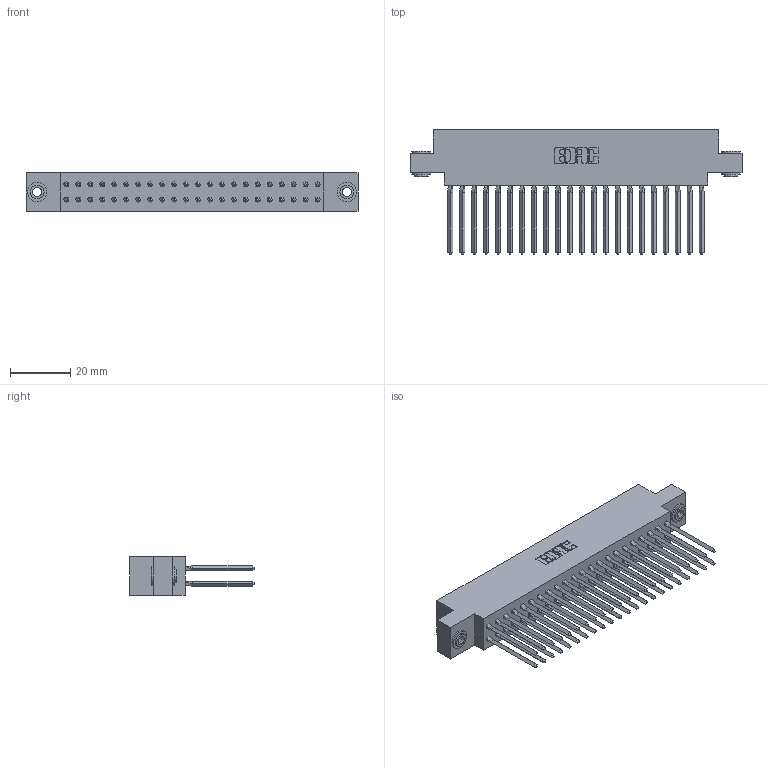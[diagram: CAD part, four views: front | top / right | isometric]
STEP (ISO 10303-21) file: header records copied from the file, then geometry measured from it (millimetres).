
FILE_DESCRIPTION (( 'STEP AP203' ), '1' );
FILE_NAME ('317-044-543-803.STEP', '2020-02-28T02:12:42', ( '' ), ( '' ), 'SwSTEP 2.0', 'SolidWorks 2016', '' );
FILE_SCHEMA (( 'CONFIG_CONTROL_DESIGN' ));
Length unit declared in the file: inch
Products named in the file (4): 317-290-001_543; 317-044-543-803; 345-250-002_345-250-002-102; 317 Part_.156 Dia - TH
Assembly tree (47 placements, depth 2):
  317-044-543-803
    317 Part_.156 Dia - TH
    317-290-001_543  x44
    345-250-002_345-250-002-102  x2
Bounding box: 109.88 x 41.15 x 12.7 mm (x, y, z)
Volume: 18003.5 mm3; surface area: 26739.4 mm2
Topology: 47 solids, 47 shells, 4056 faces, 11219 edges, 7226 vertices
Faces by surface type: plane 3280, cylinder 592, bspline 176, cone 8
Entity records: 35241 total; most frequent: CARTESIAN_POINT 6530, ORIENTED_EDGE 6022, DIRECTION 5067, EDGE_CURVE 3011, VECTOR 2731, LINE 2731, VERTEX_POINT 1999, AXIS2_PLACEMENT_3D 1168
